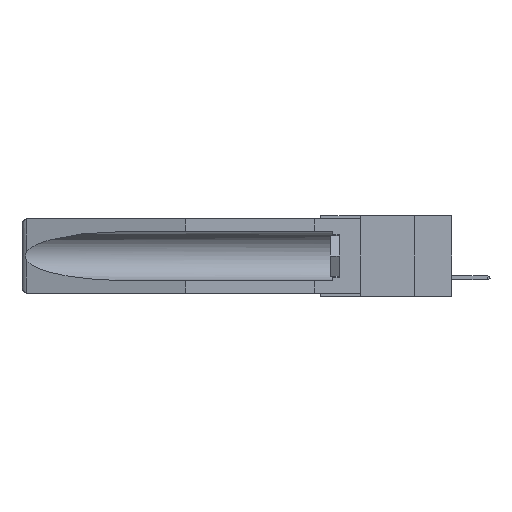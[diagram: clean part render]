
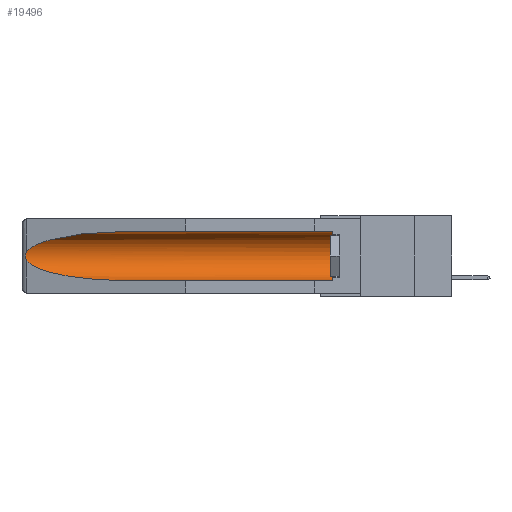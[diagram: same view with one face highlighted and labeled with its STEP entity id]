
A CAD part, left-side view. The second image highlights one B-rep face of the part: STEP entity #19496.
In plain terms, the highlighted cylindrical face has radius 2.857 mm (diameter 5.715 mm), a partial arc.
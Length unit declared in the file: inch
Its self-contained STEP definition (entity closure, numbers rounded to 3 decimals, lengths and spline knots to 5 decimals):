
#184 = CARTESIAN_POINT ( 'NONE',  ( 0.26597, 1.52961, -0.15275 ) ) ;
#259 = CARTESIAN_POINT ( 'NONE',  ( 0.2673, 1.5327, -0.16383 ) ) ;
#1088 = VERTEX_POINT ( 'NONE', #9493 ) ;
#1346 = DIRECTION ( 'NONE',  ( 0., 1., 0. ) ) ;
#1460 = CARTESIAN_POINT ( 'NONE',  ( 0.21114, 1.30732, -0.284 ) ) ;
#1904 = VERTEX_POINT ( 'NONE', #6313 ) ;
#2055 = CARTESIAN_POINT ( 'NONE',  ( 0.26655, 1.53094, -0.18657 ) ) ;
#2115 = VECTOR ( 'NONE', #1346, 39.37008 ) ;
#2139 = CARTESIAN_POINT ( 'NONE',  ( 0.2673, 1.53269, -0.17917 ) ) ;
#2292 = CARTESIAN_POINT ( 'NONE',  ( 0.155, -0.30754, -0.284 ) ) ;
#2420 = VERTEX_POINT ( 'NONE', #11699 ) ;
#3852 = CARTESIAN_POINT ( 'NONE',  ( 0.2675, 1.53308, -0.17534 ) ) ;
#4189 = EDGE_LOOP ( 'NONE', ( #14416, #18625, #7756, #8836, #14215, #16148 ) ) ;
#4803 = EDGE_CURVE ( 'NONE', #14098, #2420, #6473, .T. ) ;
#5226 = CARTESIAN_POINT ( 'NONE',  ( 0.155, -0.30754, -0.1715 ) ) ;
#5454 = FACE_OUTER_BOUND ( 'NONE', #4189, .T. ) ;
#5570 = EDGE_CURVE ( 'NONE', #8538, #1088, #12827, .T. ) ;
#5969 = CARTESIAN_POINT ( 'NONE',  ( 0.26654, 1.53092, -0.15636 ) ) ;
#6155 = CARTESIAN_POINT ( 'NONE',  ( 0.155, 1.07973, -0.059 ) ) ;
#6313 = CARTESIAN_POINT ( 'NONE',  ( 0.26537, 1.52718, -0.19328 ) ) ;
#6473 = LINE ( 'NONE', #6882, #2115 ) ;
#6882 = CARTESIAN_POINT ( 'NONE',  ( 0.155, -0.30754, -0.059 ) ) ;
#7756 = ORIENTED_EDGE ( 'NONE', *, *, #22381, .T. ) ;
#7786 = VERTEX_POINT ( 'NONE', #20561 ) ;
#7988 = CARTESIAN_POINT ( 'NONE',  ( 0.25451, 1.48313, -0.09465 ) ) ;
#8122 = CARTESIAN_POINT ( 'NONE',  ( 0.155, 0.126, -0.1715 ) ) ;
#8538 = VERTEX_POINT ( 'NONE', #16062 ) ;
#8636 = CIRCLE ( 'NONE', #24061, 0.1125 ) ;
#8739 = CARTESIAN_POINT ( 'NONE',  ( 0.155, 1.07973, -0.284 ) ) ;
#8836 = ORIENTED_EDGE ( 'NONE', *, *, #5570, .F. ) ;
#8906 = CARTESIAN_POINT ( 'NONE',  ( 0.26537, 1.52718, -0.19328 ) ) ;
#9493 = CARTESIAN_POINT ( 'NONE',  ( 0.155, 1.07973, -0.284 ) ) ;
#9824 = DIRECTION ( 'NONE',  ( 0., 1., 0. ) ) ;
#10207 = VECTOR ( 'NONE', #9824, 39.37008 ) ;
#11286 = CARTESIAN_POINT ( 'NONE',  ( 0.26537, 1.52718, -0.14972 ) ) ;
#11583 = CARTESIAN_POINT ( 'NONE',  ( 0.155, 0.126, -0.059 ) ) ;
#11699 = CARTESIAN_POINT ( 'NONE',  ( 0.155, 1.07973, -0.059 ) ) ;
#11868 = B_SPLINE_CURVE_WITH_KNOTS ( 'NONE', 3,
 ( #11286, #184, #5969, #259, #17013, #3852, #2139, #2055, #16857, #16928 ),
 .UNSPECIFIED., .F., .F.,
 ( 4, 2, 2, 2, 4 ),
 ( 0., 0.00029, 0.00058, 0.00087, 0.00117 ),
 .UNSPECIFIED. ) ;
#12718 = CYLINDRICAL_SURFACE ( 'NONE', #19962, 0.1125 ) ;
#12827 = LINE ( 'NONE', #2292, #10207 ) ;
#13320 = EDGE_CURVE ( 'NONE', #8538, #14098, #8636, .T. ) ;
#13708 = CARTESIAN_POINT ( 'NONE',  ( 0.26537, 1.52718, -0.14972 ) ) ;
#13714 = EDGE_CURVE ( 'NONE', #7786, #1904, #11868, .T. ) ;
#14004 =( BOUNDED_CURVE ( )  B_SPLINE_CURVE ( 3, ( #6155, #22938, #7988, #13708 ),
 .UNSPECIFIED., .F., .F. ) 
 B_SPLINE_CURVE_WITH_KNOTS ( ( 4, 4 ),
 ( 4.71239, 6.08839 ),
 .UNSPECIFIED. ) 
 CURVE ( )  GEOMETRIC_REPRESENTATION_ITEM ( )  RATIONAL_B_SPLINE_CURVE ( ( 1., 0.848, 0.848, 1. ) ) 
 REPRESENTATION_ITEM ( '' )  );
#14098 = VERTEX_POINT ( 'NONE', #11583 ) ;
#14215 = ORIENTED_EDGE ( 'NONE', *, *, #13320, .T. ) ;
#14416 = ORIENTED_EDGE ( 'NONE', *, *, #18325, .T. ) ;
#15645 = DIRECTION ( 'NONE',  ( 0., 0., 1. ) ) ;
#16062 = CARTESIAN_POINT ( 'NONE',  ( 0.155, 0.126, -0.284 ) ) ;
#16148 = ORIENTED_EDGE ( 'NONE', *, *, #4803, .T. ) ;
#16857 = CARTESIAN_POINT ( 'NONE',  ( 0.26597, 1.5296, -0.19026 ) ) ;
#16928 = CARTESIAN_POINT ( 'NONE',  ( 0.26537, 1.52718, -0.19328 ) ) ;
#16961 =( BOUNDED_CURVE ( )  B_SPLINE_CURVE ( 3, ( #8906, #19907, #1460, #8739 ),
 .UNSPECIFIED., .F., .F. ) 
 B_SPLINE_CURVE_WITH_KNOTS ( ( 4, 4 ),
 ( 0.1948, 1.5708 ),
 .UNSPECIFIED. ) 
 CURVE ( )  GEOMETRIC_REPRESENTATION_ITEM ( )  RATIONAL_B_SPLINE_CURVE ( ( 1., 0.848, 0.848, 1. ) ) 
 REPRESENTATION_ITEM ( '' )  );
#17013 = CARTESIAN_POINT ( 'NONE',  ( 0.2675, 1.53308, -0.16763 ) ) ;
#18226 = DIRECTION ( 'NONE',  ( 0., 1., 0. ) ) ;
#18325 = EDGE_CURVE ( 'NONE', #2420, #7786, #14004, .T. ) ;
#18625 = ORIENTED_EDGE ( 'NONE', *, *, #13714, .T. ) ;
#19496 = ADVANCED_FACE ( 'NONE', ( #5454 ), #12718, .F. ) ;
#19907 = CARTESIAN_POINT ( 'NONE',  ( 0.25451, 1.48313, -0.24835 ) ) ;
#19962 = AXIS2_PLACEMENT_3D ( 'NONE', #5226, #18226, #20330 ) ;
#20330 = DIRECTION ( 'NONE',  ( 0., 0., 1. ) ) ;
#20561 = CARTESIAN_POINT ( 'NONE',  ( 0.26537, 1.52718, -0.14972 ) ) ;
#21158 = DIRECTION ( 'NONE',  ( 0., -1., 0. ) ) ;
#22381 = EDGE_CURVE ( 'NONE', #1904, #1088, #16961, .T. ) ;
#22938 = CARTESIAN_POINT ( 'NONE',  ( 0.21114, 1.30732, -0.059 ) ) ;
#24061 = AXIS2_PLACEMENT_3D ( 'NONE', #8122, #21158, #15645 ) ;
